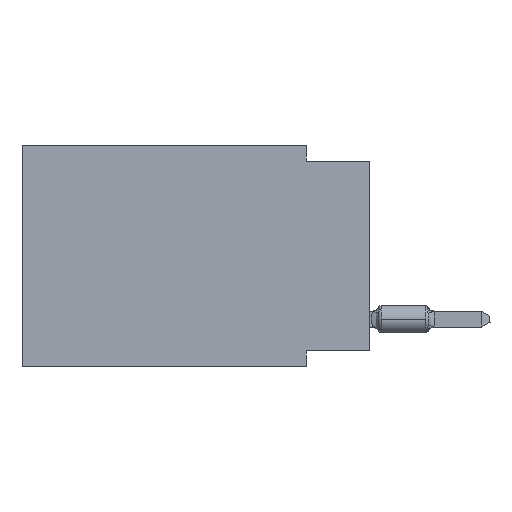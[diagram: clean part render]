
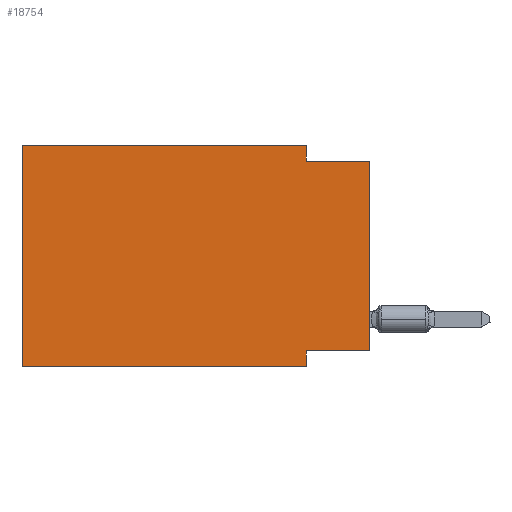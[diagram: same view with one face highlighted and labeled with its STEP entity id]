
A CAD part, left-side view. The second image highlights one B-rep face of the part: STEP entity #18754.
In plain terms, the highlighted planar face has unit normal (-1, 0, 0).
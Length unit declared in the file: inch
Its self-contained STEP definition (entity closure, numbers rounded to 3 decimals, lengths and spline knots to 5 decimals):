
#582 = DIRECTION ( 'NONE',  ( 0., -1., 0. ) ) ;
#619 = ORIENTED_EDGE ( 'NONE', *, *, #12868, .T. ) ;
#942 = DIRECTION ( 'NONE',  ( 0., 0., -1. ) ) ;
#2387 = CARTESIAN_POINT ( 'NONE',  ( 0., 0.55, -0.35 ) ) ;
#6083 = ORIENTED_EDGE ( 'NONE', *, *, #11825, .F. ) ;
#6302 = CARTESIAN_POINT ( 'NONE',  ( 0., 0.1, 0. ) ) ;
#6700 = DIRECTION ( 'NONE',  ( 0., 0., -1. ) ) ;
#6712 = VECTOR ( 'NONE', #60975, 39.37008 ) ;
#6889 = CARTESIAN_POINT ( 'NONE',  ( 0., 0.1, -0.325 ) ) ;
#7229 = EDGE_LOOP ( 'NONE', ( #619, #22613, #39656, #71942, #54826, #75409, #6083, #61906 ) ) ;
#10869 = CARTESIAN_POINT ( 'NONE',  ( 0., 0.55, 0. ) ) ;
#11292 = CARTESIAN_POINT ( 'NONE',  ( 0., 0.55, -0.35 ) ) ;
#11825 = EDGE_CURVE ( 'NONE', #17522, #12422, #62426, .T. ) ;
#12422 = VERTEX_POINT ( 'NONE', #77736 ) ;
#12613 = CARTESIAN_POINT ( 'NONE',  ( 0., 0., -0.025 ) ) ;
#12868 = EDGE_CURVE ( 'NONE', #63325, #68460, #24099, .T. ) ;
#12902 = CARTESIAN_POINT ( 'NONE',  ( 0., 0.1, -0.025 ) ) ;
#13142 = LINE ( 'NONE', #30996, #38651 ) ;
#13751 = CARTESIAN_POINT ( 'NONE',  ( 0., 0., -0.325 ) ) ;
#15642 = EDGE_CURVE ( 'NONE', #40041, #12422, #78306, .T. ) ;
#16253 = CARTESIAN_POINT ( 'NONE',  ( 0., 0.55, 0. ) ) ;
#17379 = CARTESIAN_POINT ( 'NONE',  ( 0., 0., 0. ) ) ;
#17522 = VERTEX_POINT ( 'NONE', #6889 ) ;
#17962 = EDGE_CURVE ( 'NONE', #64942, #69392, #42796, .T. ) ;
#18754 = ADVANCED_FACE ( 'NONE', ( #46994 ), #71142, .F. ) ;
#22613 = ORIENTED_EDGE ( 'NONE', *, *, #29256, .F. ) ;
#22751 = CARTESIAN_POINT ( 'NONE',  ( 0., 0., -0.025 ) ) ;
#24099 = LINE ( 'NONE', #17379, #33677 ) ;
#25107 = EDGE_CURVE ( 'NONE', #59717, #64942, #13142, .T. ) ;
#25504 = VECTOR ( 'NONE', #37961, 39.37008 ) ;
#26802 = CARTESIAN_POINT ( 'NONE',  ( 0., 0.1, 0. ) ) ;
#27226 = EDGE_CURVE ( 'NONE', #63325, #17522, #54609, .T. ) ;
#29256 = EDGE_CURVE ( 'NONE', #69392, #68460, #44731, .T. ) ;
#30996 = CARTESIAN_POINT ( 'NONE',  ( 0., 0.55, 0. ) ) ;
#31921 = EDGE_CURVE ( 'NONE', #40041, #59717, #41633, .T. ) ;
#33677 = VECTOR ( 'NONE', #58632, 39.37008 ) ;
#34110 = DIRECTION ( 'NONE',  ( 0., 0., 1. ) ) ;
#34672 = VECTOR ( 'NONE', #34110, 39.37008 ) ;
#37368 = CARTESIAN_POINT ( 'NONE',  ( 0., 0., -0.325 ) ) ;
#37961 = DIRECTION ( 'NONE',  ( 0., 1., 0. ) ) ;
#38651 = VECTOR ( 'NONE', #55175, 39.37008 ) ;
#39033 = DIRECTION ( 'NONE',  ( 0., 0., -1. ) ) ;
#39656 = ORIENTED_EDGE ( 'NONE', *, *, #17962, .F. ) ;
#40041 = VERTEX_POINT ( 'NONE', #2387 ) ;
#41633 = LINE ( 'NONE', #16253, #34672 ) ;
#42796 = LINE ( 'NONE', #6302, #57029 ) ;
#44731 = LINE ( 'NONE', #12613, #6712 ) ;
#45563 = AXIS2_PLACEMENT_3D ( 'NONE', #10869, #59261, #942 ) ;
#46994 = FACE_OUTER_BOUND ( 'NONE', #7229, .T. ) ;
#54609 = LINE ( 'NONE', #13751, #25504 ) ;
#54826 = ORIENTED_EDGE ( 'NONE', *, *, #31921, .F. ) ;
#55175 = DIRECTION ( 'NONE',  ( 0., -1., 0. ) ) ;
#55310 = CARTESIAN_POINT ( 'NONE',  ( 0., 0.1, -0.35 ) ) ;
#57029 = VECTOR ( 'NONE', #6700, 39.37008 ) ;
#57221 = VECTOR ( 'NONE', #39033, 39.37008 ) ;
#58632 = DIRECTION ( 'NONE',  ( 0., 0., 1. ) ) ;
#58651 = CARTESIAN_POINT ( 'NONE',  ( 0., 0.55, 0. ) ) ;
#59261 = DIRECTION ( 'NONE',  ( 1., 0., 0. ) ) ;
#59717 = VERTEX_POINT ( 'NONE', #58651 ) ;
#60975 = DIRECTION ( 'NONE',  ( 0., -1., 0. ) ) ;
#61906 = ORIENTED_EDGE ( 'NONE', *, *, #27226, .F. ) ;
#62426 = LINE ( 'NONE', #55310, #57221 ) ;
#63325 = VERTEX_POINT ( 'NONE', #37368 ) ;
#64942 = VERTEX_POINT ( 'NONE', #26802 ) ;
#68460 = VERTEX_POINT ( 'NONE', #22751 ) ;
#69392 = VERTEX_POINT ( 'NONE', #12902 ) ;
#71142 = PLANE ( 'NONE',  #45563 ) ;
#71942 = ORIENTED_EDGE ( 'NONE', *, *, #25107, .F. ) ;
#74530 = VECTOR ( 'NONE', #582, 39.37008 ) ;
#75409 = ORIENTED_EDGE ( 'NONE', *, *, #15642, .T. ) ;
#77736 = CARTESIAN_POINT ( 'NONE',  ( 0., 0.1, -0.35 ) ) ;
#78306 = LINE ( 'NONE', #11292, #74530 ) ;
